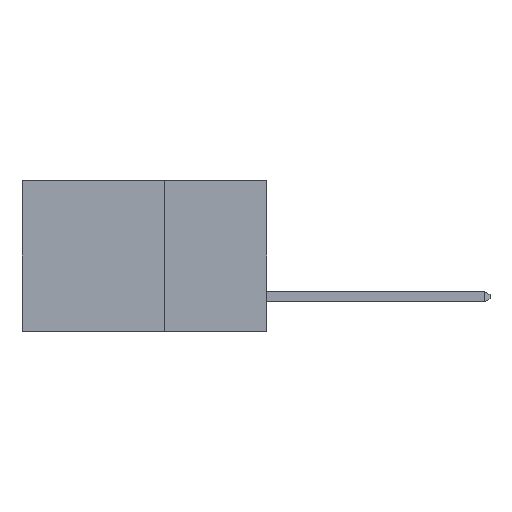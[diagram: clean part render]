
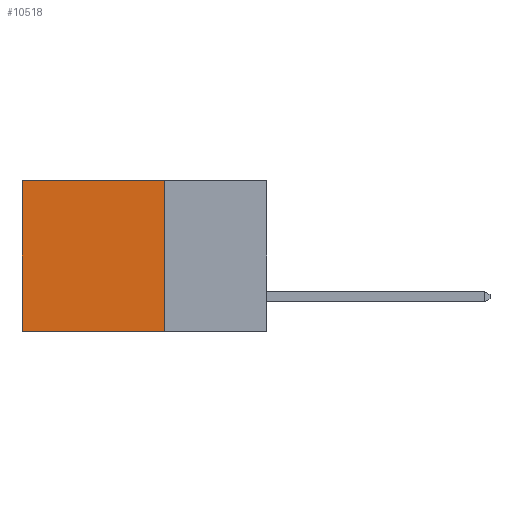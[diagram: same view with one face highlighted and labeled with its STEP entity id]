
A CAD part, left-side view. The second image highlights one B-rep face of the part: STEP entity #10518.
In plain terms, the highlighted planar face has unit normal (-1, 0, 0).
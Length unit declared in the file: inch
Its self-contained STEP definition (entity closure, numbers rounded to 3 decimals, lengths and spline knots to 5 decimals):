
#26 = VERTEX_POINT ( 'NONE', #11773 ) ;
#354 = ORIENTED_EDGE ( 'NONE', *, *, #1836, .F. ) ;
#418 = LINE ( 'NONE', #3253, #3118 ) ;
#1505 = CARTESIAN_POINT ( 'NONE',  ( 0.2875, 0.6, 0. ) ) ;
#1836 = EDGE_CURVE ( 'NONE', #5853, #26, #418, .T. ) ;
#2074 = DIRECTION ( 'NONE',  ( 0., 0., -1. ) ) ;
#2109 = EDGE_LOOP ( 'NONE', ( #10026, #354, #7924, #11072 ) ) ;
#2169 = CARTESIAN_POINT ( 'NONE',  ( 0.2875, 0.25, 0. ) ) ;
#2994 = CARTESIAN_POINT ( 'NONE',  ( 0.2875, 0.25, 0. ) ) ;
#3118 = VECTOR ( 'NONE', #7236, 39.37008 ) ;
#3253 = CARTESIAN_POINT ( 'NONE',  ( 0.2875, 0.25, -0.37 ) ) ;
#3449 = EDGE_CURVE ( 'NONE', #8324, #26, #5108, .T. ) ;
#3484 = LINE ( 'NONE', #8216, #6205 ) ;
#4092 = LINE ( 'NONE', #2169, #6917 ) ;
#4637 = CARTESIAN_POINT ( 'NONE',  ( 0.2875, 0.6, 0. ) ) ;
#5108 = LINE ( 'NONE', #1505, #8873 ) ;
#5133 = EDGE_CURVE ( 'NONE', #7717, #8324, #4092, .T. ) ;
#5376 = CARTESIAN_POINT ( 'NONE',  ( 0.2875, 0.25, -0.37 ) ) ;
#5419 = DIRECTION ( 'NONE',  ( 0., 0., -1. ) ) ;
#5853 = VERTEX_POINT ( 'NONE', #5376 ) ;
#6205 = VECTOR ( 'NONE', #5419, 39.37008 ) ;
#6917 = VECTOR ( 'NONE', #11453, 39.37008 ) ;
#7236 = DIRECTION ( 'NONE',  ( 0., 1., 0. ) ) ;
#7717 = VERTEX_POINT ( 'NONE', #9955 ) ;
#7793 = DIRECTION ( 'NONE',  ( 1., 0., 0. ) ) ;
#7852 = EDGE_CURVE ( 'NONE', #7717, #5853, #3484, .T. ) ;
#7924 = ORIENTED_EDGE ( 'NONE', *, *, #7852, .F. ) ;
#8216 = CARTESIAN_POINT ( 'NONE',  ( 0.2875, 0.25, 0. ) ) ;
#8324 = VERTEX_POINT ( 'NONE', #4637 ) ;
#8873 = VECTOR ( 'NONE', #8958, 39.37008 ) ;
#8951 = AXIS2_PLACEMENT_3D ( 'NONE', #2994, #7793, #2074 ) ;
#8958 = DIRECTION ( 'NONE',  ( 0., 0., -1. ) ) ;
#9955 = CARTESIAN_POINT ( 'NONE',  ( 0.2875, 0.25, 0. ) ) ;
#10026 = ORIENTED_EDGE ( 'NONE', *, *, #3449, .T. ) ;
#10518 = ADVANCED_FACE ( 'NONE', ( #10592 ), #10767, .F. ) ;
#10592 = FACE_OUTER_BOUND ( 'NONE', #2109, .T. ) ;
#10767 = PLANE ( 'NONE',  #8951 ) ;
#11072 = ORIENTED_EDGE ( 'NONE', *, *, #5133, .T. ) ;
#11453 = DIRECTION ( 'NONE',  ( 0., 1., 0. ) ) ;
#11773 = CARTESIAN_POINT ( 'NONE',  ( 0.2875, 0.6, -0.37 ) ) ;
